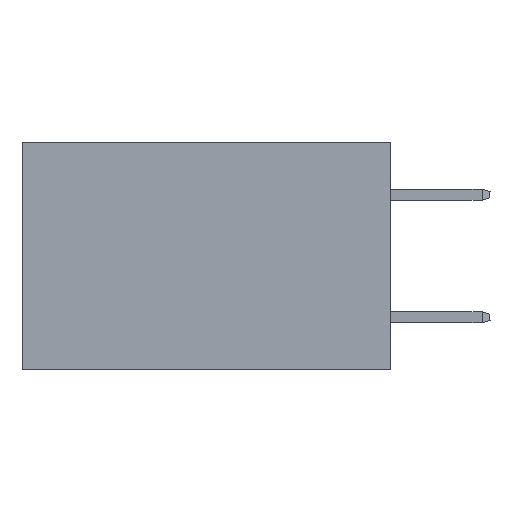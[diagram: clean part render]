
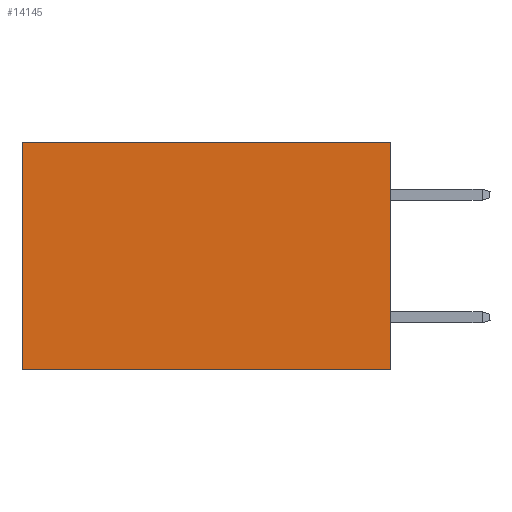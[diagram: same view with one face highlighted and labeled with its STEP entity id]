
A CAD part, left-side view. The second image highlights one B-rep face of the part: STEP entity #14145.
In plain terms, the highlighted planar face has unit normal (-1, 0, 0).
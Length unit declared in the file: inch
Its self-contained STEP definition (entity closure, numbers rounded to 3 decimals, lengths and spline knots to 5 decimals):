
#828 = VERTEX_POINT ( 'NONE', #39187 ) ;
#1986 = VERTEX_POINT ( 'NONE', #14029 ) ;
#2306 = DIRECTION ( 'NONE',  ( 0., 0., -1. ) ) ;
#3025 = VERTEX_POINT ( 'NONE', #33867 ) ;
#3247 = EDGE_CURVE ( 'NONE', #11355, #828, #3979, .T. ) ;
#3248 = ORIENTED_EDGE ( 'NONE', *, *, #21545, .F. ) ;
#3979 = LINE ( 'NONE', #32219, #35289 ) ;
#4072 = LINE ( 'NONE', #37004, #9183 ) ;
#4150 = ORIENTED_EDGE ( 'NONE', *, *, #3247, .T. ) ;
#4463 = EDGE_LOOP ( 'NONE', ( #4150, #25375, #3248, #24942 ) ) ;
#5228 = EDGE_CURVE ( 'NONE', #3025, #11355, #35612, .T. ) ;
#7670 = CARTESIAN_POINT ( 'NONE',  ( 0.2875, 0., 0. ) ) ;
#8916 = EDGE_CURVE ( 'NONE', #1986, #828, #4072, .T. ) ;
#9183 = VECTOR ( 'NONE', #19372, 39.37008 ) ;
#9654 = FACE_OUTER_BOUND ( 'NONE', #4463, .T. ) ;
#10667 = CARTESIAN_POINT ( 'NONE',  ( 0.2875, 0.6, 0. ) ) ;
#11355 = VERTEX_POINT ( 'NONE', #10667 ) ;
#13023 = PLANE ( 'NONE',  #17419 ) ;
#13161 = DIRECTION ( 'NONE',  ( 1., 0., 0. ) ) ;
#13910 = LINE ( 'NONE', #26271, #21061 ) ;
#14029 = CARTESIAN_POINT ( 'NONE',  ( 0.2875, 0., -0.37 ) ) ;
#14145 = ADVANCED_FACE ( 'NONE', ( #9654 ), #13023, .F. ) ;
#17419 = AXIS2_PLACEMENT_3D ( 'NONE', #19076, #13161, #22113 ) ;
#19076 = CARTESIAN_POINT ( 'NONE',  ( 0.2875, 0., 0. ) ) ;
#19372 = DIRECTION ( 'NONE',  ( 0., 1., 0. ) ) ;
#21061 = VECTOR ( 'NONE', #2306, 39.37008 ) ;
#21545 = EDGE_CURVE ( 'NONE', #3025, #1986, #13910, .T. ) ;
#22113 = DIRECTION ( 'NONE',  ( 0., 0., -1. ) ) ;
#24216 = VECTOR ( 'NONE', #25878, 39.37008 ) ;
#24942 = ORIENTED_EDGE ( 'NONE', *, *, #5228, .T. ) ;
#25375 = ORIENTED_EDGE ( 'NONE', *, *, #8916, .F. ) ;
#25878 = DIRECTION ( 'NONE',  ( 0., 1., 0. ) ) ;
#26271 = CARTESIAN_POINT ( 'NONE',  ( 0.2875, 0., 0. ) ) ;
#32219 = CARTESIAN_POINT ( 'NONE',  ( 0.2875, 0.6, 0. ) ) ;
#32985 = DIRECTION ( 'NONE',  ( 0., 0., -1. ) ) ;
#33867 = CARTESIAN_POINT ( 'NONE',  ( 0.2875, 0., 0. ) ) ;
#35289 = VECTOR ( 'NONE', #32985, 39.37008 ) ;
#35612 = LINE ( 'NONE', #7670, #24216 ) ;
#37004 = CARTESIAN_POINT ( 'NONE',  ( 0.2875, 0., -0.37 ) ) ;
#39187 = CARTESIAN_POINT ( 'NONE',  ( 0.2875, 0.6, -0.37 ) ) ;
